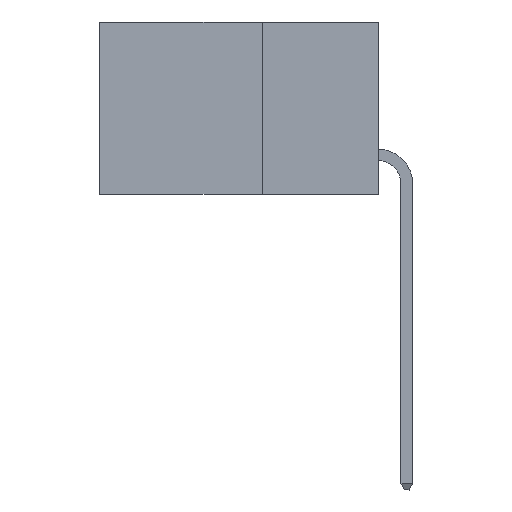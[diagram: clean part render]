
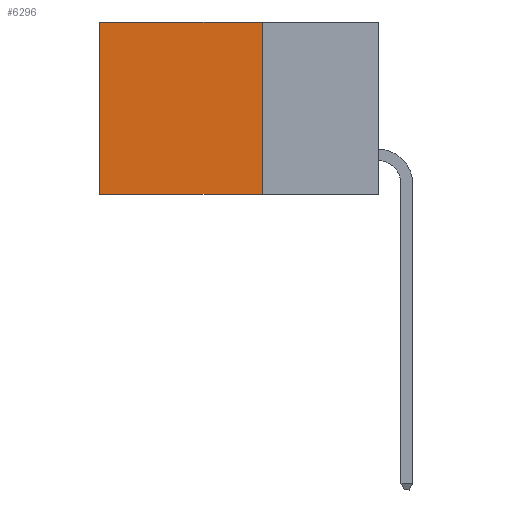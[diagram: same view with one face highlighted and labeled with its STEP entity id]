
A CAD part, left-side view. The second image highlights one B-rep face of the part: STEP entity #6296.
In plain terms, the highlighted planar face has unit normal (-1, 0, 0).
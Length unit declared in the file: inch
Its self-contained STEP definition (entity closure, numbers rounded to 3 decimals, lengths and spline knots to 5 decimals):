
#2 = EDGE_CURVE ( 'NONE', #4294, #1726, #14369, .T. ) ;
#728 = VERTEX_POINT ( 'NONE', #9045 ) ;
#1683 = VECTOR ( 'NONE', #10887, 39.37008 ) ;
#1726 = VERTEX_POINT ( 'NONE', #14647 ) ;
#2057 = EDGE_LOOP ( 'NONE', ( #15426, #3929, #3518, #6666 ) ) ;
#3440 = DIRECTION ( 'NONE',  ( 0., 0., -1. ) ) ;
#3484 = EDGE_CURVE ( 'NONE', #728, #8488, #9464, .T. ) ;
#3518 = ORIENTED_EDGE ( 'NONE', *, *, #2, .F. ) ;
#3929 = ORIENTED_EDGE ( 'NONE', *, *, #8641, .F. ) ;
#4294 = VERTEX_POINT ( 'NONE', #6795 ) ;
#4507 = LINE ( 'NONE', #20342, #1683 ) ;
#5152 = CARTESIAN_POINT ( 'NONE',  ( 0.2615, 0.6, -0.37 ) ) ;
#5756 = LINE ( 'NONE', #20036, #8693 ) ;
#6221 = AXIS2_PLACEMENT_3D ( 'NONE', #17955, #8546, #14846 ) ;
#6296 = ADVANCED_FACE ( 'NONE', ( #13165 ), #19498, .F. ) ;
#6406 = CARTESIAN_POINT ( 'NONE',  ( 0.2615, 0.25, -0.37 ) ) ;
#6666 = ORIENTED_EDGE ( 'NONE', *, *, #11533, .T. ) ;
#6795 = CARTESIAN_POINT ( 'NONE',  ( 0.2615, 0.25, 0. ) ) ;
#8488 = VERTEX_POINT ( 'NONE', #5152 ) ;
#8546 = DIRECTION ( 'NONE',  ( 1., 0., 0. ) ) ;
#8641 = EDGE_CURVE ( 'NONE', #1726, #8488, #4507, .T. ) ;
#8693 = VECTOR ( 'NONE', #16632, 39.37008 ) ;
#9045 = CARTESIAN_POINT ( 'NONE',  ( 0.2615, 0.6, 0. ) ) ;
#9464 = LINE ( 'NONE', #14217, #10592 ) ;
#10592 = VECTOR ( 'NONE', #3440, 39.37008 ) ;
#10887 = DIRECTION ( 'NONE',  ( 0., 1., 0. ) ) ;
#11436 = VECTOR ( 'NONE', #19044, 39.37008 ) ;
#11533 = EDGE_CURVE ( 'NONE', #4294, #728, #5756, .T. ) ;
#13165 = FACE_OUTER_BOUND ( 'NONE', #2057, .T. ) ;
#14217 = CARTESIAN_POINT ( 'NONE',  ( 0.2615, 0.6, -0.37 ) ) ;
#14369 = LINE ( 'NONE', #6406, #11436 ) ;
#14647 = CARTESIAN_POINT ( 'NONE',  ( 0.2615, 0.25, -0.37 ) ) ;
#14846 = DIRECTION ( 'NONE',  ( 0., 0., -1. ) ) ;
#15426 = ORIENTED_EDGE ( 'NONE', *, *, #3484, .T. ) ;
#16632 = DIRECTION ( 'NONE',  ( 0., 1., 0. ) ) ;
#17955 = CARTESIAN_POINT ( 'NONE',  ( 0.2615, 0.25, -0.37 ) ) ;
#19044 = DIRECTION ( 'NONE',  ( 0., 0., -1. ) ) ;
#19498 = PLANE ( 'NONE',  #6221 ) ;
#20036 = CARTESIAN_POINT ( 'NONE',  ( 0.2615, 0.25, 0. ) ) ;
#20342 = CARTESIAN_POINT ( 'NONE',  ( 0.2615, 0.25, -0.37 ) ) ;
